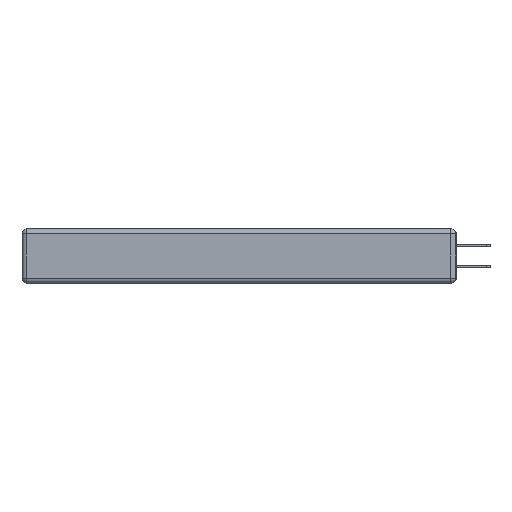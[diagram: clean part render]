
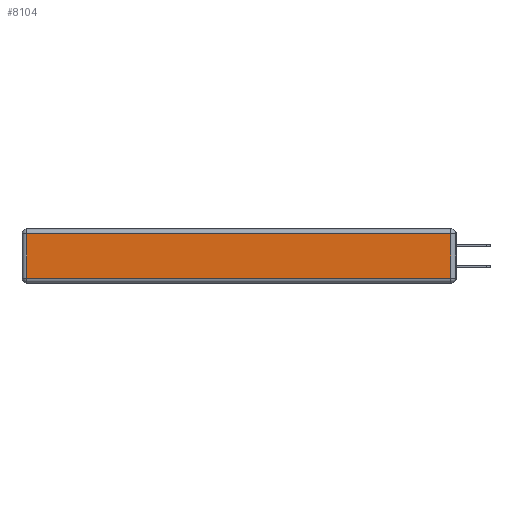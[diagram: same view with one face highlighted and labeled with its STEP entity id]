
A CAD part, left-side view. The second image highlights one B-rep face of the part: STEP entity #8104.
In plain terms, the highlighted planar face has unit normal (-1, 0, 0).
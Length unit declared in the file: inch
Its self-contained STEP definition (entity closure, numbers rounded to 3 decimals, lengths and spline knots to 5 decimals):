
#909 = VECTOR ( 'NONE', #1603, 39.37008 ) ;
#1110 = DIRECTION ( 'NONE',  ( 0., 0., 1. ) ) ;
#1603 = DIRECTION ( 'NONE',  ( 0., 0., -1. ) ) ;
#2182 = CARTESIAN_POINT ( 'NONE',  ( 0., 0.03, -0.343 ) ) ;
#2328 = DIRECTION ( 'NONE',  ( 0., 1., 0. ) ) ;
#2481 = VERTEX_POINT ( 'NONE', #12154 ) ;
#3047 = AXIS2_PLACEMENT_3D ( 'NONE', #8877, #11045, #5400 ) ;
#3261 = EDGE_CURVE ( 'NONE', #10493, #12234, #6131, .T. ) ;
#4132 = CARTESIAN_POINT ( 'NONE',  ( 0., 2.72, -0.03 ) ) ;
#4174 = DIRECTION ( 'NONE',  ( 0., -1., 0. ) ) ;
#4215 = EDGE_CURVE ( 'NONE', #8808, #2481, #12773, .T. ) ;
#5400 = DIRECTION ( 'NONE',  ( 0., 0., 1. ) ) ;
#5597 = VECTOR ( 'NONE', #2328, 39.37008 ) ;
#6103 = FACE_OUTER_BOUND ( 'NONE', #9896, .T. ) ;
#6131 = LINE ( 'NONE', #7941, #5597 ) ;
#7131 = LINE ( 'NONE', #2182, #10265 ) ;
#7941 = CARTESIAN_POINT ( 'NONE',  ( 0., 2.75, -0.03 ) ) ;
#7954 = CARTESIAN_POINT ( 'NONE',  ( 0., 2.72, -0.313 ) ) ;
#8104 = ADVANCED_FACE ( 'NONE', ( #6103 ), #13411, .T. ) ;
#8253 = CARTESIAN_POINT ( 'NONE',  ( 0., 2.72, -0.343 ) ) ;
#8616 = ORIENTED_EDGE ( 'NONE', *, *, #13630, .T. ) ;
#8808 = VERTEX_POINT ( 'NONE', #7954 ) ;
#8877 = CARTESIAN_POINT ( 'NONE',  ( 0., 0., -0.343 ) ) ;
#8880 = CARTESIAN_POINT ( 'NONE',  ( 0., 0.03, -0.03 ) ) ;
#9593 = ORIENTED_EDGE ( 'NONE', *, *, #4215, .T. ) ;
#9797 = LINE ( 'NONE', #8253, #909 ) ;
#9872 = EDGE_CURVE ( 'NONE', #2481, #10493, #7131, .T. ) ;
#9896 = EDGE_LOOP ( 'NONE', ( #9593, #14313, #11145, #8616 ) ) ;
#10265 = VECTOR ( 'NONE', #1110, 39.37008 ) ;
#10286 = VECTOR ( 'NONE', #4174, 39.37008 ) ;
#10493 = VERTEX_POINT ( 'NONE', #8880 ) ;
#11009 = CARTESIAN_POINT ( 'NONE',  ( 0., 0., -0.313 ) ) ;
#11045 = DIRECTION ( 'NONE',  ( -1., 0., 0. ) ) ;
#11145 = ORIENTED_EDGE ( 'NONE', *, *, #3261, .T. ) ;
#12154 = CARTESIAN_POINT ( 'NONE',  ( 0., 0.03, -0.313 ) ) ;
#12234 = VERTEX_POINT ( 'NONE', #4132 ) ;
#12773 = LINE ( 'NONE', #11009, #10286 ) ;
#13411 = PLANE ( 'NONE',  #3047 ) ;
#13630 = EDGE_CURVE ( 'NONE', #12234, #8808, #9797, .T. ) ;
#14313 = ORIENTED_EDGE ( 'NONE', *, *, #9872, .T. ) ;
